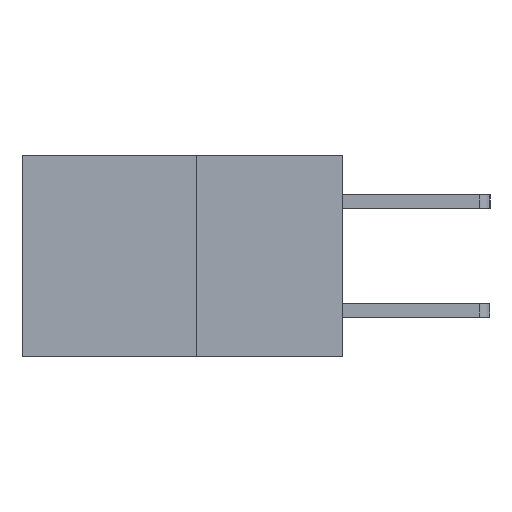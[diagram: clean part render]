
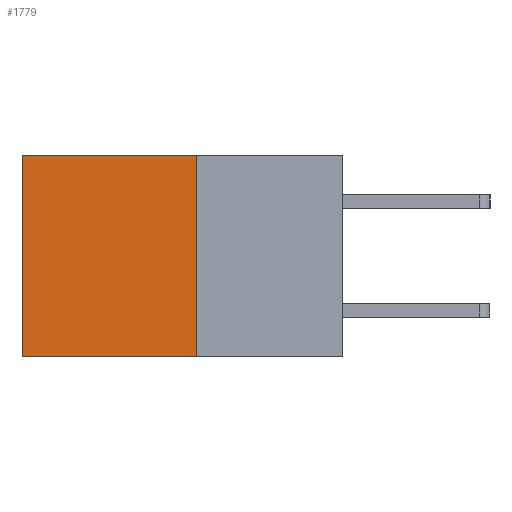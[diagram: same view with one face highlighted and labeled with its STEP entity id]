
A CAD part, left-side view. The second image highlights one B-rep face of the part: STEP entity #1779.
In plain terms, the highlighted planar face has unit normal (-1, 0, 0).
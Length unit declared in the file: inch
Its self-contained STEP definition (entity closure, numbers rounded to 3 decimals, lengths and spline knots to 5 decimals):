
#41 = VERTEX_POINT ( 'NONE', #7291 ) ;
#188 = VECTOR ( 'NONE', #2102, 39.37008 ) ;
#448 = VERTEX_POINT ( 'NONE', #4840 ) ;
#658 = ORIENTED_EDGE ( 'NONE', *, *, #4527, .T. ) ;
#755 = ORIENTED_EDGE ( 'NONE', *, *, #1015, .F. ) ;
#787 = ORIENTED_EDGE ( 'NONE', *, *, #1609, .F. ) ;
#867 = ORIENTED_EDGE ( 'NONE', *, *, #7946, .T. ) ;
#1015 = EDGE_CURVE ( 'NONE', #9760, #41, #9751, .T. ) ;
#1609 = EDGE_CURVE ( 'NONE', #3666, #9760, #11023, .T. ) ;
#1779 = ADVANCED_FACE ( 'NONE', ( #4471 ), #8944, .F. ) ;
#2102 = DIRECTION ( 'NONE',  ( 0., 1., 0. ) ) ;
#2408 = CARTESIAN_POINT ( 'NONE',  ( 0.277, 0.27, 0. ) ) ;
#2633 = CARTESIAN_POINT ( 'NONE',  ( 0.277, 0.59, -0.37 ) ) ;
#3310 = DIRECTION ( 'NONE',  ( 0., 0., -1. ) ) ;
#3666 = VERTEX_POINT ( 'NONE', #6113 ) ;
#4135 = CARTESIAN_POINT ( 'NONE',  ( 0.277, 0.27, -0.37 ) ) ;
#4403 = EDGE_LOOP ( 'NONE', ( #658, #755, #787, #867 ) ) ;
#4471 = FACE_OUTER_BOUND ( 'NONE', #4403, .T. ) ;
#4527 = EDGE_CURVE ( 'NONE', #448, #41, #9807, .T. ) ;
#4702 = VECTOR ( 'NONE', #3310, 39.37008 ) ;
#4840 = CARTESIAN_POINT ( 'NONE',  ( 0.277, 0.59, 0. ) ) ;
#4886 = CARTESIAN_POINT ( 'NONE',  ( 0.277, 0.27, -0.37 ) ) ;
#5476 = LINE ( 'NONE', #2408, #10264 ) ;
#5518 = AXIS2_PLACEMENT_3D ( 'NONE', #6157, #7627, #11851 ) ;
#6113 = CARTESIAN_POINT ( 'NONE',  ( 0.277, 0.27, 0. ) ) ;
#6157 = CARTESIAN_POINT ( 'NONE',  ( 0.277, 0.27, -0.37 ) ) ;
#7291 = CARTESIAN_POINT ( 'NONE',  ( 0.277, 0.59, -0.37 ) ) ;
#7627 = DIRECTION ( 'NONE',  ( 1., 0., 0. ) ) ;
#7946 = EDGE_CURVE ( 'NONE', #3666, #448, #5476, .T. ) ;
#8267 = VECTOR ( 'NONE', #12516, 39.37008 ) ;
#8305 = DIRECTION ( 'NONE',  ( 0., 1., 0. ) ) ;
#8944 = PLANE ( 'NONE',  #5518 ) ;
#9501 = CARTESIAN_POINT ( 'NONE',  ( 0.277, 0.27, -0.37 ) ) ;
#9751 = LINE ( 'NONE', #9501, #188 ) ;
#9760 = VERTEX_POINT ( 'NONE', #4135 ) ;
#9807 = LINE ( 'NONE', #2633, #4702 ) ;
#10264 = VECTOR ( 'NONE', #8305, 39.37008 ) ;
#11023 = LINE ( 'NONE', #4886, #8267 ) ;
#11851 = DIRECTION ( 'NONE',  ( 0., 0., -1. ) ) ;
#12516 = DIRECTION ( 'NONE',  ( 0., 0., -1. ) ) ;
